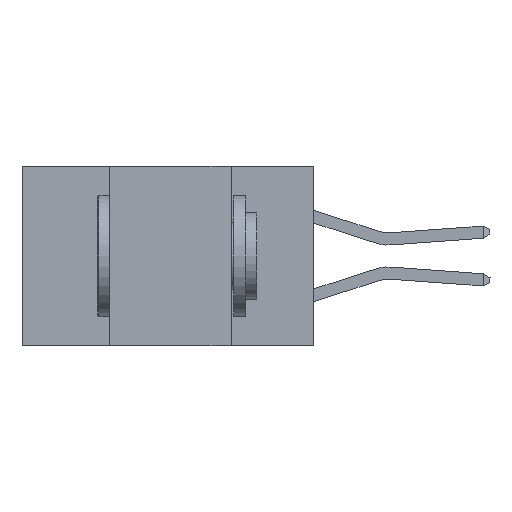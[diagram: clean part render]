
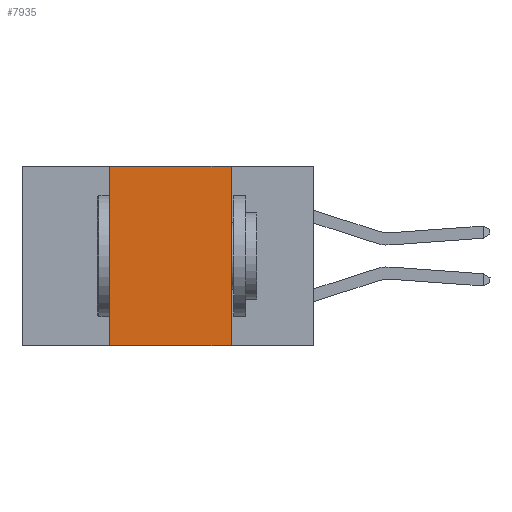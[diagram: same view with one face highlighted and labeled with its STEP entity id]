
A CAD part, left-side view. The second image highlights one B-rep face of the part: STEP entity #7935.
In plain terms, the highlighted planar face has unit normal (-1, 0, 0).
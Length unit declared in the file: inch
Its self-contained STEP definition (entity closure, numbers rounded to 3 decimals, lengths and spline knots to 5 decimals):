
#591 = CARTESIAN_POINT ( 'NONE',  ( 0., 0.42, 0. ) ) ;
#931 = PLANE ( 'NONE',  #23814 ) ;
#974 = EDGE_CURVE ( 'NONE', #14335, #9602, #25671, .T. ) ;
#1767 = CARTESIAN_POINT ( 'NONE',  ( 0., 0.17, 0. ) ) ;
#1907 = EDGE_CURVE ( 'NONE', #26660, #23961, #8303, .T. ) ;
#4051 = LINE ( 'NONE', #591, #9066 ) ;
#5093 = DIRECTION ( 'NONE',  ( 0., 0., -1. ) ) ;
#6884 = DIRECTION ( 'NONE',  ( 0., -1., 0. ) ) ;
#7935 = ADVANCED_FACE ( 'NONE', ( #20154 ), #931, .F. ) ;
#8303 = LINE ( 'NONE', #13518, #19228 ) ;
#8328 = CARTESIAN_POINT ( 'NONE',  ( 0., 0.42, -0.37 ) ) ;
#8510 = CARTESIAN_POINT ( 'NONE',  ( 0., 0.6, -0.37 ) ) ;
#9066 = VECTOR ( 'NONE', #25216, 39.37008 ) ;
#9248 = DIRECTION ( 'NONE',  ( 0., 0., -1. ) ) ;
#9602 = VERTEX_POINT ( 'NONE', #27729 ) ;
#10362 = ORIENTED_EDGE ( 'NONE', *, *, #1907, .F. ) ;
#10987 = EDGE_CURVE ( 'NONE', #14335, #26660, #4051, .T. ) ;
#11696 = CARTESIAN_POINT ( 'NONE',  ( 0., 0.17, 0. ) ) ;
#13518 = CARTESIAN_POINT ( 'NONE',  ( 0., 0.6, 0. ) ) ;
#14335 = VERTEX_POINT ( 'NONE', #8328 ) ;
#14710 = VECTOR ( 'NONE', #9248, 39.37008 ) ;
#16112 = ORIENTED_EDGE ( 'NONE', *, *, #10987, .F. ) ;
#16366 = DIRECTION ( 'NONE',  ( 1., 0., 0. ) ) ;
#18658 = CARTESIAN_POINT ( 'NONE',  ( 0., 0.6, 0. ) ) ;
#18864 = EDGE_CURVE ( 'NONE', #23961, #9602, #21726, .T. ) ;
#19228 = VECTOR ( 'NONE', #6884, 39.37008 ) ;
#20089 = ORIENTED_EDGE ( 'NONE', *, *, #974, .T. ) ;
#20154 = FACE_OUTER_BOUND ( 'NONE', #27018, .T. ) ;
#20364 = ORIENTED_EDGE ( 'NONE', *, *, #18864, .F. ) ;
#21726 = LINE ( 'NONE', #11696, #14710 ) ;
#22108 = VECTOR ( 'NONE', #22680, 39.37008 ) ;
#22680 = DIRECTION ( 'NONE',  ( 0., -1., 0. ) ) ;
#23814 = AXIS2_PLACEMENT_3D ( 'NONE', #18658, #16366, #5093 ) ;
#23961 = VERTEX_POINT ( 'NONE', #1767 ) ;
#24896 = CARTESIAN_POINT ( 'NONE',  ( 0., 0.42, 0. ) ) ;
#25216 = DIRECTION ( 'NONE',  ( 0., 0., 1. ) ) ;
#25671 = LINE ( 'NONE', #8510, #22108 ) ;
#26660 = VERTEX_POINT ( 'NONE', #24896 ) ;
#27018 = EDGE_LOOP ( 'NONE', ( #20364, #10362, #16112, #20089 ) ) ;
#27729 = CARTESIAN_POINT ( 'NONE',  ( 0., 0.17, -0.37 ) ) ;
